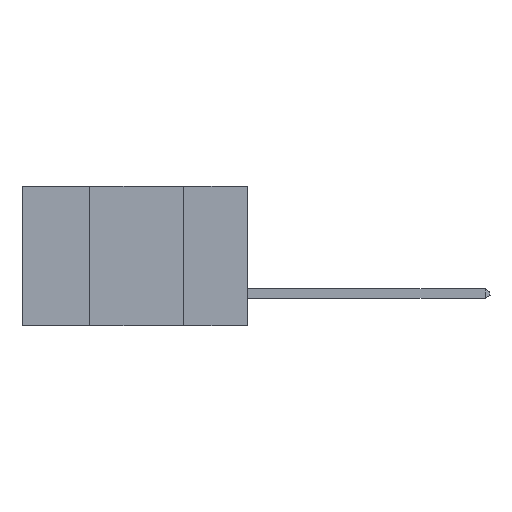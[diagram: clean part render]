
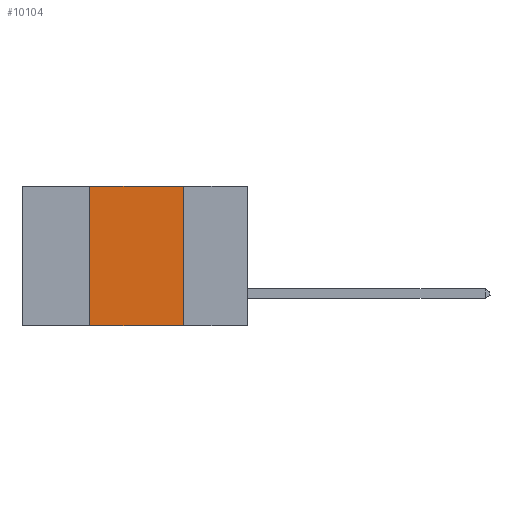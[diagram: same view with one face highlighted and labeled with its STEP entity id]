
A CAD part, left-side view. The second image highlights one B-rep face of the part: STEP entity #10104.
In plain terms, the highlighted planar face has unit normal (-1, 0, 0).
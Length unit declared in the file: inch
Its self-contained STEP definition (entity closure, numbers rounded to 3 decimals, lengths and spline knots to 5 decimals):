
#511 = VECTOR ( 'NONE', #7435, 39.37008 ) ;
#855 = DIRECTION ( 'NONE',  ( 0., 0., -1. ) ) ;
#1295 = CARTESIAN_POINT ( 'NONE',  ( 0., 0.6, -0.37 ) ) ;
#1317 = CARTESIAN_POINT ( 'NONE',  ( 0., 0.42, 0. ) ) ;
#2679 = VECTOR ( 'NONE', #3733, 39.37008 ) ;
#3733 = DIRECTION ( 'NONE',  ( 0., 0., -1. ) ) ;
#4052 = FACE_OUTER_BOUND ( 'NONE', #17198, .T. ) ;
#4597 = EDGE_CURVE ( 'NONE', #8988, #17912, #16213, .T. ) ;
#6239 = DIRECTION ( 'NONE',  ( 0., 0., 1. ) ) ;
#6978 = ORIENTED_EDGE ( 'NONE', *, *, #4597, .F. ) ;
#7435 = DIRECTION ( 'NONE',  ( 0., -1., 0. ) ) ;
#7484 = LINE ( 'NONE', #1295, #11326 ) ;
#8255 = CARTESIAN_POINT ( 'NONE',  ( 0., 0.17, 0. ) ) ;
#8631 = CARTESIAN_POINT ( 'NONE',  ( 0., 0.17, -0.37 ) ) ;
#8948 = CARTESIAN_POINT ( 'NONE',  ( 0., 0.42, -0.37 ) ) ;
#8950 = LINE ( 'NONE', #13120, #13942 ) ;
#8988 = VERTEX_POINT ( 'NONE', #1317 ) ;
#9235 = EDGE_CURVE ( 'NONE', #17912, #15799, #12055, .T. ) ;
#9667 = AXIS2_PLACEMENT_3D ( 'NONE', #15001, #9850, #855 ) ;
#9850 = DIRECTION ( 'NONE',  ( 1., 0., 0. ) ) ;
#9924 = DIRECTION ( 'NONE',  ( 0., -1., 0. ) ) ;
#10038 = ORIENTED_EDGE ( 'NONE', *, *, #9235, .F. ) ;
#10104 = ADVANCED_FACE ( 'NONE', ( #4052 ), #18319, .F. ) ;
#10152 = EDGE_CURVE ( 'NONE', #12223, #8988, #8950, .T. ) ;
#11107 = EDGE_CURVE ( 'NONE', #12223, #15799, #7484, .T. ) ;
#11326 = VECTOR ( 'NONE', #9924, 39.37008 ) ;
#12055 = LINE ( 'NONE', #12818, #2679 ) ;
#12223 = VERTEX_POINT ( 'NONE', #8948 ) ;
#12818 = CARTESIAN_POINT ( 'NONE',  ( 0., 0.17, 0. ) ) ;
#13120 = CARTESIAN_POINT ( 'NONE',  ( 0., 0.42, 0. ) ) ;
#13942 = VECTOR ( 'NONE', #6239, 39.37008 ) ;
#15001 = CARTESIAN_POINT ( 'NONE',  ( 0., 0.6, 0. ) ) ;
#15231 = ORIENTED_EDGE ( 'NONE', *, *, #11107, .T. ) ;
#15799 = VERTEX_POINT ( 'NONE', #8631 ) ;
#16213 = LINE ( 'NONE', #19825, #511 ) ;
#17198 = EDGE_LOOP ( 'NONE', ( #10038, #6978, #17799, #15231 ) ) ;
#17799 = ORIENTED_EDGE ( 'NONE', *, *, #10152, .F. ) ;
#17912 = VERTEX_POINT ( 'NONE', #8255 ) ;
#18319 = PLANE ( 'NONE',  #9667 ) ;
#19825 = CARTESIAN_POINT ( 'NONE',  ( 0., 0.6, 0. ) ) ;
